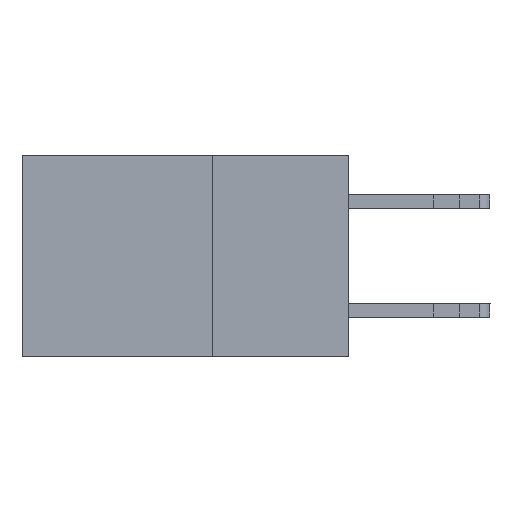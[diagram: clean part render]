
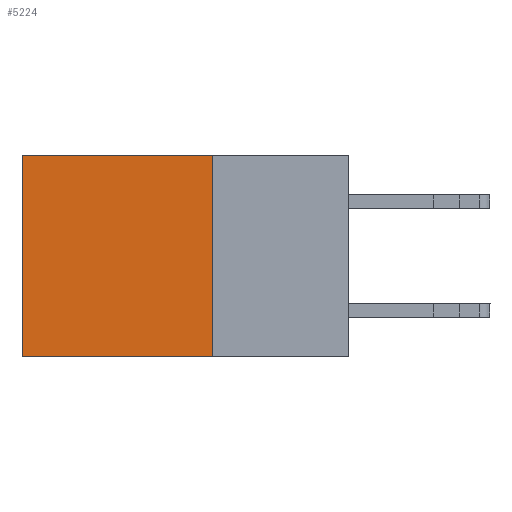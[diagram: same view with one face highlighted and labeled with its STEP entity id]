
A CAD part, left-side view. The second image highlights one B-rep face of the part: STEP entity #5224.
In plain terms, the highlighted planar face has unit normal (-1, 0, 0).
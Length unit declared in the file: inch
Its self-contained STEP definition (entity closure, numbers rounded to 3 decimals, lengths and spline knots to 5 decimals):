
#50 = DIRECTION ( 'NONE',  ( 0., 1., 0. ) ) ;
#138 = EDGE_CURVE ( 'NONE', #9243, #669, #9777, .T. ) ;
#188 = CARTESIAN_POINT ( 'NONE',  ( 0.2615, 0.25, -0.37 ) ) ;
#669 = VERTEX_POINT ( 'NONE', #2794 ) ;
#1169 = DIRECTION ( 'NONE',  ( 1., 0., 0. ) ) ;
#1810 = EDGE_CURVE ( 'NONE', #9029, #669, #4968, .T. ) ;
#2647 = VECTOR ( 'NONE', #8670, 39.37008 ) ;
#2794 = CARTESIAN_POINT ( 'NONE',  ( 0.2615, 0.6, -0.37 ) ) ;
#2845 = ORIENTED_EDGE ( 'NONE', *, *, #1810, .F. ) ;
#3454 = DIRECTION ( 'NONE',  ( 0., 0., -1. ) ) ;
#3504 = CARTESIAN_POINT ( 'NONE',  ( 0.2615, 0.25, 0. ) ) ;
#3659 = VECTOR ( 'NONE', #3454, 39.37008 ) ;
#3959 = LINE ( 'NONE', #188, #3659 ) ;
#4306 = CARTESIAN_POINT ( 'NONE',  ( 0.2615, 0.25, -0.37 ) ) ;
#4598 = VECTOR ( 'NONE', #6103, 39.37008 ) ;
#4844 = LINE ( 'NONE', #3504, #4598 ) ;
#4968 = LINE ( 'NONE', #4306, #11242 ) ;
#5224 = ADVANCED_FACE ( 'NONE', ( #9694 ), #10809, .F. ) ;
#5324 = EDGE_CURVE ( 'NONE', #10573, #9029, #3959, .T. ) ;
#5515 = ORIENTED_EDGE ( 'NONE', *, *, #10221, .T. ) ;
#5905 = CARTESIAN_POINT ( 'NONE',  ( 0.2615, 0.25, -0.37 ) ) ;
#6017 = AXIS2_PLACEMENT_3D ( 'NONE', #5905, #1169, #7628 ) ;
#6103 = DIRECTION ( 'NONE',  ( 0., 1., 0. ) ) ;
#6350 = CARTESIAN_POINT ( 'NONE',  ( 0.2615, 0.6, 0. ) ) ;
#7510 = ORIENTED_EDGE ( 'NONE', *, *, #5324, .F. ) ;
#7628 = DIRECTION ( 'NONE',  ( 0., 0., -1. ) ) ;
#8670 = DIRECTION ( 'NONE',  ( 0., 0., -1. ) ) ;
#8730 = CARTESIAN_POINT ( 'NONE',  ( 0.2615, 0.25, -0.37 ) ) ;
#9029 = VERTEX_POINT ( 'NONE', #8730 ) ;
#9243 = VERTEX_POINT ( 'NONE', #6350 ) ;
#9424 = ORIENTED_EDGE ( 'NONE', *, *, #138, .T. ) ;
#9694 = FACE_OUTER_BOUND ( 'NONE', #11407, .T. ) ;
#9777 = LINE ( 'NONE', #10857, #2647 ) ;
#10221 = EDGE_CURVE ( 'NONE', #10573, #9243, #4844, .T. ) ;
#10401 = CARTESIAN_POINT ( 'NONE',  ( 0.2615, 0.25, 0. ) ) ;
#10573 = VERTEX_POINT ( 'NONE', #10401 ) ;
#10809 = PLANE ( 'NONE',  #6017 ) ;
#10857 = CARTESIAN_POINT ( 'NONE',  ( 0.2615, 0.6, -0.37 ) ) ;
#11242 = VECTOR ( 'NONE', #50, 39.37008 ) ;
#11407 = EDGE_LOOP ( 'NONE', ( #9424, #2845, #7510, #5515 ) ) ;
